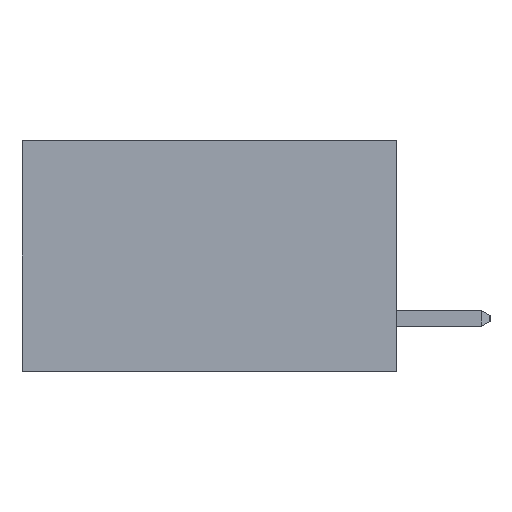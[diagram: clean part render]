
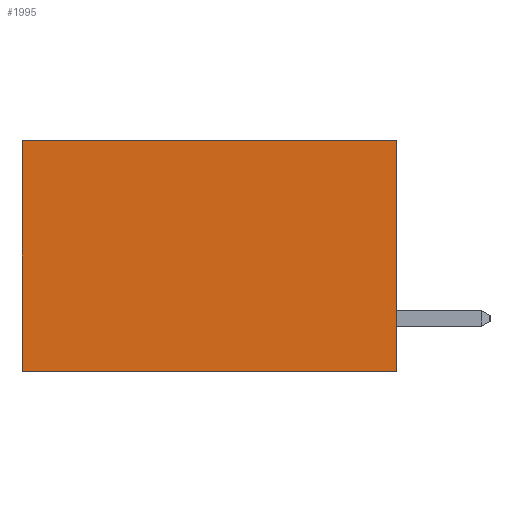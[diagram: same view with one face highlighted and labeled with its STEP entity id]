
A CAD part, left-side view. The second image highlights one B-rep face of the part: STEP entity #1995.
In plain terms, the highlighted planar face has unit normal (-1, 0, 0).
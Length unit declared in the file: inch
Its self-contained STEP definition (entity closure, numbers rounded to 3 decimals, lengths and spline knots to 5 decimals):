
#697 = LINE ( 'NONE', #17845, #20598 ) ;
#833 = CARTESIAN_POINT ( 'NONE',  ( 0.298, 0., 0. ) ) ;
#1075 = LINE ( 'NONE', #13489, #11329 ) ;
#1501 = CARTESIAN_POINT ( 'NONE',  ( 0.298, 0., -0.37 ) ) ;
#1860 = CARTESIAN_POINT ( 'NONE',  ( 0.298, 0., -0.37 ) ) ;
#1927 = DIRECTION ( 'NONE',  ( 0., 1., 0. ) ) ;
#1995 = ADVANCED_FACE ( 'NONE', ( #9369 ), #5893, .F. ) ;
#2381 = ORIENTED_EDGE ( 'NONE', *, *, #22554, .T. ) ;
#2940 = ORIENTED_EDGE ( 'NONE', *, *, #3517, .F. ) ;
#3517 = EDGE_CURVE ( 'NONE', #14927, #20001, #3845, .T. ) ;
#3845 = LINE ( 'NONE', #1501, #12872 ) ;
#4601 = EDGE_LOOP ( 'NONE', ( #6790, #2940, #19279, #2381 ) ) ;
#5568 = CARTESIAN_POINT ( 'NONE',  ( 0.298, 0., 0. ) ) ;
#5618 = CARTESIAN_POINT ( 'NONE',  ( 0.298, 0., 0. ) ) ;
#5893 = PLANE ( 'NONE',  #21673 ) ;
#6790 = ORIENTED_EDGE ( 'NONE', *, *, #9177, .T. ) ;
#9177 = EDGE_CURVE ( 'NONE', #20065, #20001, #697, .T. ) ;
#9369 = FACE_OUTER_BOUND ( 'NONE', #4601, .T. ) ;
#11329 = VECTOR ( 'NONE', #1927, 39.37008 ) ;
#11645 = DIRECTION ( 'NONE',  ( 0., 0., -1. ) ) ;
#12463 = CARTESIAN_POINT ( 'NONE',  ( 0.298, 0.6, 0. ) ) ;
#12872 = VECTOR ( 'NONE', #18821, 39.37008 ) ;
#13103 = DIRECTION ( 'NONE',  ( 1., 0., 0. ) ) ;
#13489 = CARTESIAN_POINT ( 'NONE',  ( 0.298, 0., 0. ) ) ;
#14927 = VERTEX_POINT ( 'NONE', #1860 ) ;
#16364 = VECTOR ( 'NONE', #24624, 39.37008 ) ;
#17845 = CARTESIAN_POINT ( 'NONE',  ( 0.298, 0.6, 0. ) ) ;
#18045 = CARTESIAN_POINT ( 'NONE',  ( 0.298, 0.6, -0.37 ) ) ;
#18821 = DIRECTION ( 'NONE',  ( 0., 1., 0. ) ) ;
#19279 = ORIENTED_EDGE ( 'NONE', *, *, #20237, .F. ) ;
#19755 = DIRECTION ( 'NONE',  ( 0., 0., -1. ) ) ;
#20001 = VERTEX_POINT ( 'NONE', #18045 ) ;
#20065 = VERTEX_POINT ( 'NONE', #12463 ) ;
#20237 = EDGE_CURVE ( 'NONE', #23166, #14927, #21419, .T. ) ;
#20598 = VECTOR ( 'NONE', #19755, 39.37008 ) ;
#21419 = LINE ( 'NONE', #5568, #16364 ) ;
#21673 = AXIS2_PLACEMENT_3D ( 'NONE', #833, #13103, #11645 ) ;
#22554 = EDGE_CURVE ( 'NONE', #23166, #20065, #1075, .T. ) ;
#23166 = VERTEX_POINT ( 'NONE', #5618 ) ;
#24624 = DIRECTION ( 'NONE',  ( 0., 0., -1. ) ) ;
